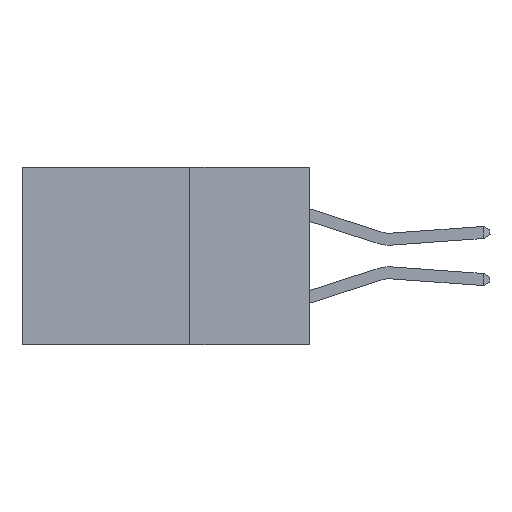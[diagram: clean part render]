
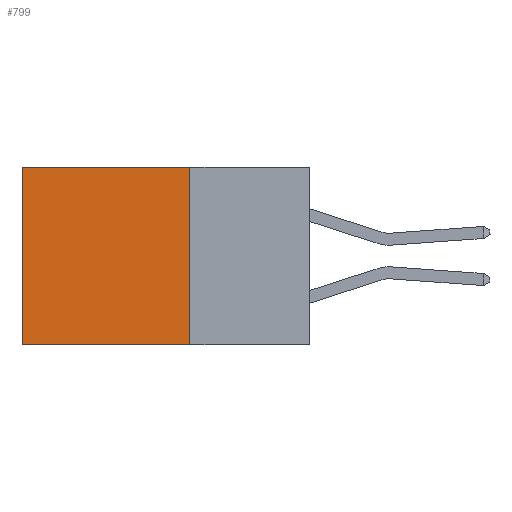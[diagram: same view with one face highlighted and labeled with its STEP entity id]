
A CAD part, left-side view. The second image highlights one B-rep face of the part: STEP entity #799.
In plain terms, the highlighted planar face has unit normal (-1, 0, 0).
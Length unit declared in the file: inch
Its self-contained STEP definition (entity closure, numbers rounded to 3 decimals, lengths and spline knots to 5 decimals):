
#611 = ORIENTED_EDGE ( 'NONE', *, *, #2937, .T. ) ;
#739 = VECTOR ( 'NONE', #8592, 39.37008 ) ;
#749 = CARTESIAN_POINT ( 'NONE',  ( 0.2615, 0.25, 0. ) ) ;
#799 = ADVANCED_FACE ( 'NONE', ( #1327 ), #2110, .F. ) ;
#1092 = VERTEX_POINT ( 'NONE', #6309 ) ;
#1112 = ORIENTED_EDGE ( 'NONE', *, *, #3715, .F. ) ;
#1285 = AXIS2_PLACEMENT_3D ( 'NONE', #3389, #1943, #5821 ) ;
#1327 = FACE_OUTER_BOUND ( 'NONE', #4494, .T. ) ;
#1834 = ORIENTED_EDGE ( 'NONE', *, *, #2707, .T. ) ;
#1943 = DIRECTION ( 'NONE',  ( 1., 0., 0. ) ) ;
#2110 = PLANE ( 'NONE',  #1285 ) ;
#2401 = VERTEX_POINT ( 'NONE', #5268 ) ;
#2695 = DIRECTION ( 'NONE',  ( 0., 1., 0. ) ) ;
#2707 = EDGE_CURVE ( 'NONE', #3477, #1092, #5020, .T. ) ;
#2937 = EDGE_CURVE ( 'NONE', #1092, #2401, #3332, .T. ) ;
#3061 = DIRECTION ( 'NONE',  ( 0., 1., 0. ) ) ;
#3332 = LINE ( 'NONE', #6177, #4788 ) ;
#3389 = CARTESIAN_POINT ( 'NONE',  ( 0.2615, 0.25, -0.37 ) ) ;
#3477 = VERTEX_POINT ( 'NONE', #3747 ) ;
#3715 = EDGE_CURVE ( 'NONE', #8357, #2401, #6773, .T. ) ;
#3747 = CARTESIAN_POINT ( 'NONE',  ( 0.2615, 0.25, 0. ) ) ;
#4494 = EDGE_LOOP ( 'NONE', ( #611, #1112, #4884, #1834 ) ) ;
#4501 = EDGE_CURVE ( 'NONE', #3477, #8357, #6182, .T. ) ;
#4788 = VECTOR ( 'NONE', #6766, 39.37008 ) ;
#4859 = CARTESIAN_POINT ( 'NONE',  ( 0.2615, 0.25, -0.37 ) ) ;
#4884 = ORIENTED_EDGE ( 'NONE', *, *, #4501, .F. ) ;
#5020 = LINE ( 'NONE', #749, #7978 ) ;
#5268 = CARTESIAN_POINT ( 'NONE',  ( 0.2615, 0.6, -0.37 ) ) ;
#5723 = CARTESIAN_POINT ( 'NONE',  ( 0.2615, 0.25, -0.37 ) ) ;
#5821 = DIRECTION ( 'NONE',  ( 0., 0., -1. ) ) ;
#6177 = CARTESIAN_POINT ( 'NONE',  ( 0.2615, 0.6, -0.37 ) ) ;
#6182 = LINE ( 'NONE', #5723, #739 ) ;
#6309 = CARTESIAN_POINT ( 'NONE',  ( 0.2615, 0.6, 0. ) ) ;
#6586 = VECTOR ( 'NONE', #2695, 39.37008 ) ;
#6766 = DIRECTION ( 'NONE',  ( 0., 0., -1. ) ) ;
#6773 = LINE ( 'NONE', #4859, #6586 ) ;
#7680 = CARTESIAN_POINT ( 'NONE',  ( 0.2615, 0.25, -0.37 ) ) ;
#7978 = VECTOR ( 'NONE', #3061, 39.37008 ) ;
#8357 = VERTEX_POINT ( 'NONE', #7680 ) ;
#8592 = DIRECTION ( 'NONE',  ( 0., 0., -1. ) ) ;
